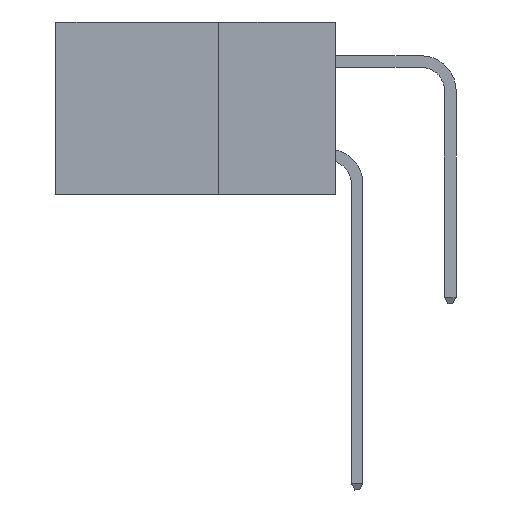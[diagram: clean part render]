
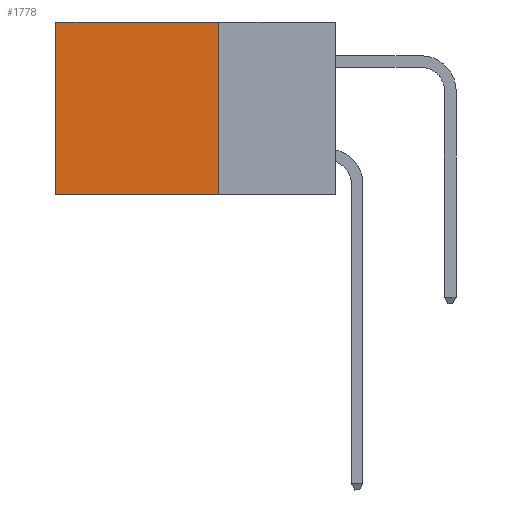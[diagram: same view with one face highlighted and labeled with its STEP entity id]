
A CAD part, left-side view. The second image highlights one B-rep face of the part: STEP entity #1778.
In plain terms, the highlighted planar face has unit normal (-1, 0, 0).
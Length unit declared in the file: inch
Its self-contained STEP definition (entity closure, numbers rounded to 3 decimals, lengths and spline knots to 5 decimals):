
#449 = VECTOR ( 'NONE', #18298, 39.37008 ) ;
#531 = EDGE_CURVE ( 'NONE', #17299, #10183, #19295, .T. ) ;
#1504 = EDGE_LOOP ( 'NONE', ( #10641, #6865, #3774, #7696 ) ) ;
#1778 = ADVANCED_FACE ( 'NONE', ( #19250 ), #2626, .F. ) ;
#2232 = CARTESIAN_POINT ( 'NONE',  ( 0.2875, 0.25, -0.37 ) ) ;
#2260 = AXIS2_PLACEMENT_3D ( 'NONE', #15040, #19432, #13277 ) ;
#2626 = PLANE ( 'NONE',  #2260 ) ;
#2687 = VECTOR ( 'NONE', #3736, 39.37008 ) ;
#2920 = LINE ( 'NONE', #14824, #18895 ) ;
#3122 = LINE ( 'NONE', #24779, #449 ) ;
#3291 = CARTESIAN_POINT ( 'NONE',  ( 0.2875, 0.6, -0.37 ) ) ;
#3736 = DIRECTION ( 'NONE',  ( 0., 1., 0. ) ) ;
#3774 = ORIENTED_EDGE ( 'NONE', *, *, #25029, .F. ) ;
#6865 = ORIENTED_EDGE ( 'NONE', *, *, #531, .F. ) ;
#7572 = CARTESIAN_POINT ( 'NONE',  ( 0.2875, 0.25, -0.37 ) ) ;
#7696 = ORIENTED_EDGE ( 'NONE', *, *, #17643, .T. ) ;
#10183 = VERTEX_POINT ( 'NONE', #3291 ) ;
#10641 = ORIENTED_EDGE ( 'NONE', *, *, #20991, .T. ) ;
#12014 = VECTOR ( 'NONE', #14064, 39.37008 ) ;
#13020 = VERTEX_POINT ( 'NONE', #20245 ) ;
#13277 = DIRECTION ( 'NONE',  ( 0., 0., -1. ) ) ;
#14064 = DIRECTION ( 'NONE',  ( 0., 0., -1. ) ) ;
#14824 = CARTESIAN_POINT ( 'NONE',  ( 0.2875, 0.25, 0. ) ) ;
#15040 = CARTESIAN_POINT ( 'NONE',  ( 0.2875, 0.25, 0. ) ) ;
#16414 = CARTESIAN_POINT ( 'NONE',  ( 0.2875, 0.25, 0. ) ) ;
#17299 = VERTEX_POINT ( 'NONE', #2232 ) ;
#17643 = EDGE_CURVE ( 'NONE', #13020, #23968, #2920, .T. ) ;
#18298 = DIRECTION ( 'NONE',  ( 0., 0., -1. ) ) ;
#18895 = VECTOR ( 'NONE', #23123, 39.37008 ) ;
#19250 = FACE_OUTER_BOUND ( 'NONE', #1504, .T. ) ;
#19295 = LINE ( 'NONE', #7572, #2687 ) ;
#19432 = DIRECTION ( 'NONE',  ( 1., 0., 0. ) ) ;
#20245 = CARTESIAN_POINT ( 'NONE',  ( 0.2875, 0.25, 0. ) ) ;
#20991 = EDGE_CURVE ( 'NONE', #23968, #10183, #3122, .T. ) ;
#22361 = LINE ( 'NONE', #16414, #12014 ) ;
#23123 = DIRECTION ( 'NONE',  ( 0., 1., 0. ) ) ;
#23968 = VERTEX_POINT ( 'NONE', #25819 ) ;
#24779 = CARTESIAN_POINT ( 'NONE',  ( 0.2875, 0.6, 0. ) ) ;
#25029 = EDGE_CURVE ( 'NONE', #13020, #17299, #22361, .T. ) ;
#25819 = CARTESIAN_POINT ( 'NONE',  ( 0.2875, 0.6, 0. ) ) ;
